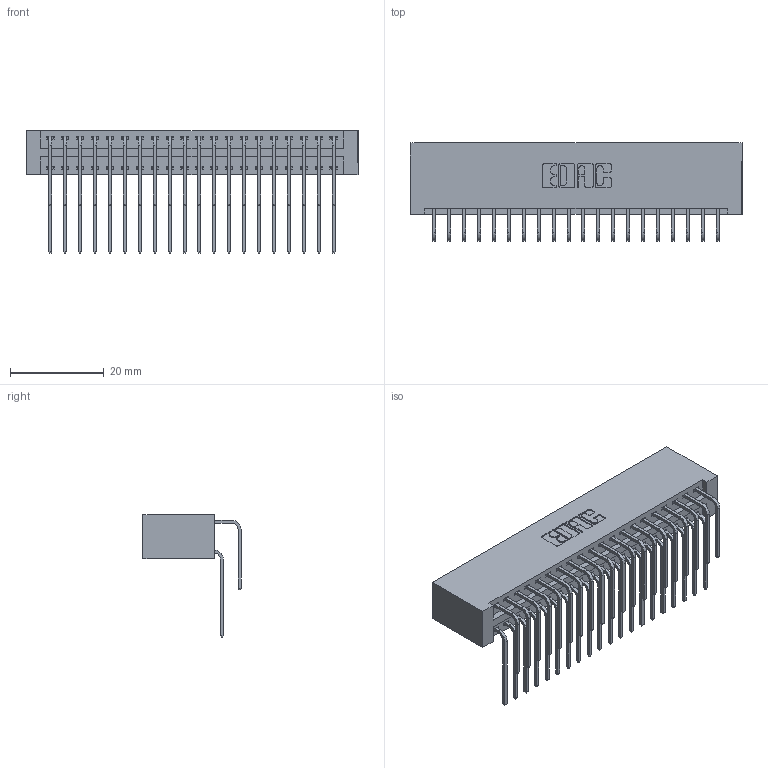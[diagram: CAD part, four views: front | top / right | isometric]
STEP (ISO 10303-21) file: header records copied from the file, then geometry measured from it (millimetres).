
FILE_DESCRIPTION (( 'STEP AP203' ), '1' );
FILE_NAME ('396-040-559-201.STEP', '2019-11-03T07:30:52', ( '' ), ( '' ), 'SwSTEP 2.0', 'SolidWorks 2016', '' );
FILE_SCHEMA (( 'CONFIG_CONTROL_DESIGN' ));
Length unit declared in the file: inch
Products named in the file (4): 345-292-001_559 Tail - 2; 345-292-001_558 559 Tail - 1; 346 Part_No Mounting Lugs; 396-040-559-201
Assembly tree (41 placements, depth 2):
  396-040-559-201
    346 Part_No Mounting Lugs
    345-292-001_558 559 Tail - 1  x20
    345-292-001_559 Tail - 2  x20
Bounding box: 70.74 x 20.89 x 26.16 mm (x, y, z)
Volume: 7531.1 mm3; surface area: 11276.4 mm2
Topology: 41 solids, 41 shells, 2274 faces, 6745 edges, 4442 vertices
Faces by surface type: plane 1552, cylinder 722
Entity records: 17521 total; most frequent: CARTESIAN_POINT 2967, ORIENTED_EDGE 2850, DIRECTION 2633, EDGE_CURVE 1425, VECTOR 1181, LINE 1181, VERTEX_POINT 946, AXIS2_PLACEMENT_3D 726
